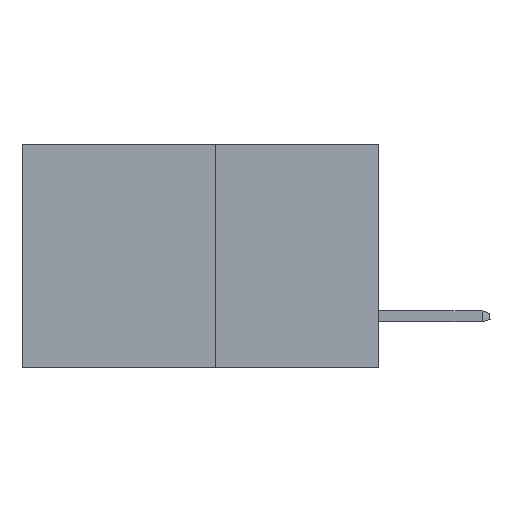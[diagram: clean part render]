
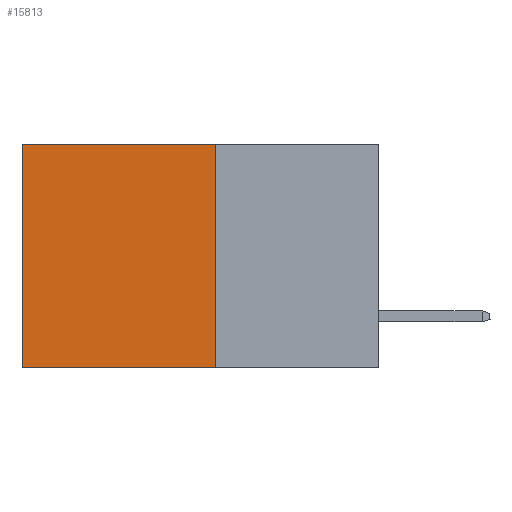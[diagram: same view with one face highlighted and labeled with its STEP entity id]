
A CAD part, left-side view. The second image highlights one B-rep face of the part: STEP entity #15813.
In plain terms, the highlighted planar face has unit normal (-1, 0, 0).
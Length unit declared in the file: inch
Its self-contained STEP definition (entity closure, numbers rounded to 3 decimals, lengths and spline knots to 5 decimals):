
#332 = VECTOR ( 'NONE', #1312, 39.37008 ) ;
#680 = CARTESIAN_POINT ( 'NONE',  ( 0.277, 0.27, -0.37 ) ) ;
#1071 = LINE ( 'NONE', #10974, #7704 ) ;
#1312 = DIRECTION ( 'NONE',  ( 0., 0., -1. ) ) ;
#1413 = CARTESIAN_POINT ( 'NONE',  ( 0.277, 0.59, -0.37 ) ) ;
#1933 = EDGE_CURVE ( 'NONE', #6418, #16341, #12017, .T. ) ;
#2233 = EDGE_CURVE ( 'NONE', #16341, #15289, #13733, .T. ) ;
#2273 = VECTOR ( 'NONE', #2681, 39.37008 ) ;
#2321 = EDGE_CURVE ( 'NONE', #6418, #10841, #1071, .T. ) ;
#2369 = CARTESIAN_POINT ( 'NONE',  ( 0.277, 0.27, 0. ) ) ;
#2650 = FACE_OUTER_BOUND ( 'NONE', #14601, .T. ) ;
#2681 = DIRECTION ( 'NONE',  ( 0., 1., 0. ) ) ;
#3941 = LINE ( 'NONE', #680, #12367 ) ;
#4834 = CARTESIAN_POINT ( 'NONE',  ( 0.277, 0.27, -0.37 ) ) ;
#5968 = ORIENTED_EDGE ( 'NONE', *, *, #2233, .T. ) ;
#6056 = ORIENTED_EDGE ( 'NONE', *, *, #14200, .F. ) ;
#6060 = ORIENTED_EDGE ( 'NONE', *, *, #2321, .F. ) ;
#6096 = ORIENTED_EDGE ( 'NONE', *, *, #1933, .T. ) ;
#6156 = PLANE ( 'NONE',  #14550 ) ;
#6418 = VERTEX_POINT ( 'NONE', #15799 ) ;
#7449 = DIRECTION ( 'NONE',  ( 1., 0., 0. ) ) ;
#7704 = VECTOR ( 'NONE', #15062, 39.37008 ) ;
#8613 = DIRECTION ( 'NONE',  ( 0., 1., 0. ) ) ;
#10791 = CARTESIAN_POINT ( 'NONE',  ( 0.277, 0.59, 0. ) ) ;
#10841 = VERTEX_POINT ( 'NONE', #4834 ) ;
#10974 = CARTESIAN_POINT ( 'NONE',  ( 0.277, 0.27, -0.37 ) ) ;
#12017 = LINE ( 'NONE', #2369, #2273 ) ;
#12367 = VECTOR ( 'NONE', #8613, 39.37008 ) ;
#13733 = LINE ( 'NONE', #1413, #332 ) ;
#14200 = EDGE_CURVE ( 'NONE', #10841, #15289, #3941, .T. ) ;
#14550 = AXIS2_PLACEMENT_3D ( 'NONE', #14830, #7449, #16048 ) ;
#14601 = EDGE_LOOP ( 'NONE', ( #5968, #6056, #6060, #6096 ) ) ;
#14830 = CARTESIAN_POINT ( 'NONE',  ( 0.277, 0.27, -0.37 ) ) ;
#15062 = DIRECTION ( 'NONE',  ( 0., 0., -1. ) ) ;
#15289 = VERTEX_POINT ( 'NONE', #16466 ) ;
#15799 = CARTESIAN_POINT ( 'NONE',  ( 0.277, 0.27, 0. ) ) ;
#15813 = ADVANCED_FACE ( 'NONE', ( #2650 ), #6156, .F. ) ;
#16048 = DIRECTION ( 'NONE',  ( 0., 0., -1. ) ) ;
#16341 = VERTEX_POINT ( 'NONE', #10791 ) ;
#16466 = CARTESIAN_POINT ( 'NONE',  ( 0.277, 0.59, -0.37 ) ) ;
